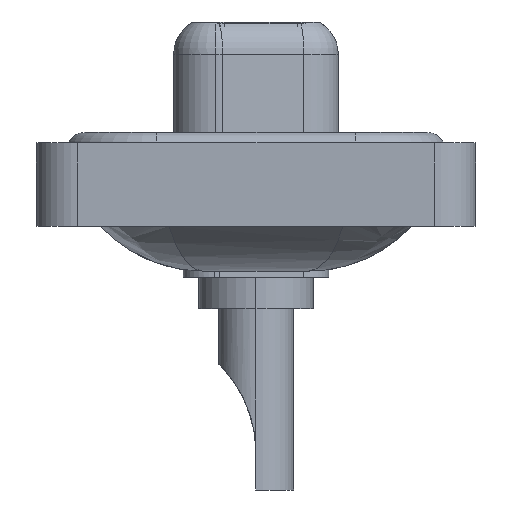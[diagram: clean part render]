
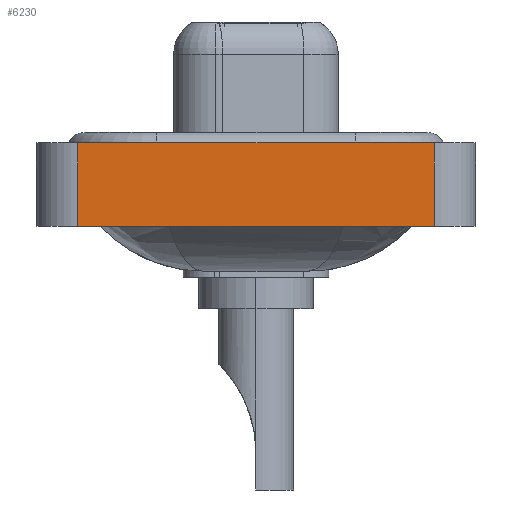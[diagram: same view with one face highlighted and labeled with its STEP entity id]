
A CAD part, left-side view. The second image highlights one B-rep face of the part: STEP entity #6230.
In plain terms, the highlighted planar face has unit normal (-1, 0, 0).
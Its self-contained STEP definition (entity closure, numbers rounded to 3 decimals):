
#739 = CARTESIAN_POINT ( 'NONE',  ( -7.35, 8.55, 0.4 ) ) ;
#844 = DIRECTION ( 'NONE',  ( 0., 0., 1. ) ) ;
#1175 = DIRECTION ( 'NONE',  ( 0., -1., 0. ) ) ;
#1421 = ORIENTED_EDGE ( 'NONE', *, *, #4559, .F. ) ;
#2042 = CARTESIAN_POINT ( 'NONE',  ( -7.35, -8.55, -3.6 ) ) ;
#2225 = EDGE_CURVE ( 'NONE', #6335, #13793, #13662, .T. ) ;
#2234 = EDGE_LOOP ( 'NONE', ( #4146, #10267, #1421, #14030 ) ) ;
#3189 = EDGE_CURVE ( 'NONE', #9028, #6335, #6481, .T. ) ;
#4146 = ORIENTED_EDGE ( 'NONE', *, *, #2225, .T. ) ;
#4257 = DIRECTION ( 'NONE',  ( 0., 0., 1. ) ) ;
#4559 = EDGE_CURVE ( 'NONE', #9028, #5020, #4836, .T. ) ;
#4836 = LINE ( 'NONE', #16474, #15609 ) ;
#5020 = VERTEX_POINT ( 'NONE', #739 ) ;
#5131 = CARTESIAN_POINT ( 'NONE',  ( -7.35, 8.55, -3.6 ) ) ;
#5569 = PLANE ( 'NONE',  #11768 ) ;
#6230 = ADVANCED_FACE ( 'NONE', ( #10856 ), #5569, .T. ) ;
#6331 = CARTESIAN_POINT ( 'NONE',  ( -7.35, -8.55, -3.6 ) ) ;
#6335 = VERTEX_POINT ( 'NONE', #12738 ) ;
#6481 = LINE ( 'NONE', #6331, #13232 ) ;
#8937 = CARTESIAN_POINT ( 'NONE',  ( -7.35, -8.55, 0.4 ) ) ;
#9028 = VERTEX_POINT ( 'NONE', #5131 ) ;
#9524 = VECTOR ( 'NONE', #1175, 1000. ) ;
#10267 = ORIENTED_EDGE ( 'NONE', *, *, #16237, .F. ) ;
#10746 = VECTOR ( 'NONE', #4257, 1000. ) ;
#10783 = CARTESIAN_POINT ( 'NONE',  ( -7.35, -8.55, -3.6 ) ) ;
#10856 = FACE_OUTER_BOUND ( 'NONE', #2234, .T. ) ;
#10972 = CARTESIAN_POINT ( 'NONE',  ( -7.35, -8.55, 0.4 ) ) ;
#11195 = DIRECTION ( 'NONE',  ( 0., 0., 1. ) ) ;
#11413 = LINE ( 'NONE', #8937, #9524 ) ;
#11768 = AXIS2_PLACEMENT_3D ( 'NONE', #10783, #12141, #11195 ) ;
#12141 = DIRECTION ( 'NONE',  ( -1., 0., 0. ) ) ;
#12738 = CARTESIAN_POINT ( 'NONE',  ( -7.35, -8.55, -3.6 ) ) ;
#13232 = VECTOR ( 'NONE', #16759, 1000. ) ;
#13662 = LINE ( 'NONE', #2042, #10746 ) ;
#13793 = VERTEX_POINT ( 'NONE', #10972 ) ;
#14030 = ORIENTED_EDGE ( 'NONE', *, *, #3189, .T. ) ;
#15609 = VECTOR ( 'NONE', #844, 1000. ) ;
#16237 = EDGE_CURVE ( 'NONE', #5020, #13793, #11413, .T. ) ;
#16474 = CARTESIAN_POINT ( 'NONE',  ( -7.35, 8.55, -3.6 ) ) ;
#16759 = DIRECTION ( 'NONE',  ( 0., -1., 0. ) ) ;
